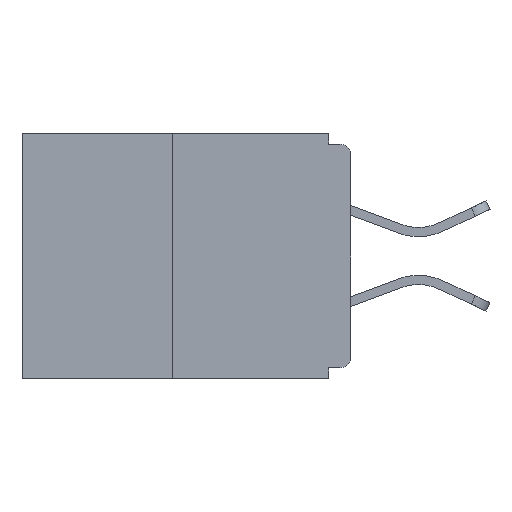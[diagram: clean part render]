
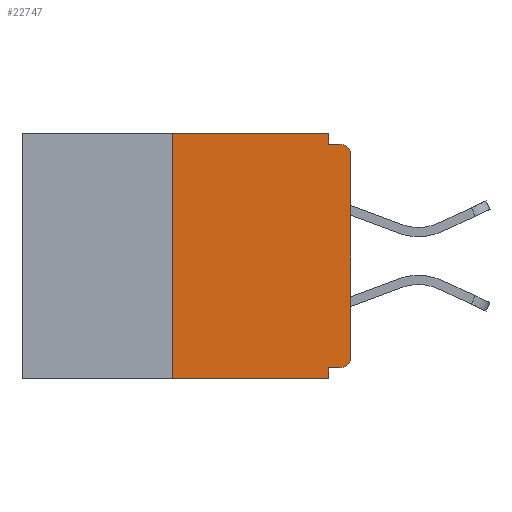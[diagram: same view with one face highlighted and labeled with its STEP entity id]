
A CAD part, left-side view. The second image highlights one B-rep face of the part: STEP entity #22747.
In plain terms, the highlighted planar face has unit normal (-1, 0, 0).
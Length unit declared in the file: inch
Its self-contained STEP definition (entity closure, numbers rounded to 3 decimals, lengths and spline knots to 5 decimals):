
#349 = EDGE_CURVE ( 'NONE', #19427, #4706, #14187, .T. ) ;
#406 = VECTOR ( 'NONE', #24897, 39.37008 ) ;
#541 = DIRECTION ( 'NONE',  ( 0., 0., -1. ) ) ;
#572 = EDGE_CURVE ( 'NONE', #20106, #1014, #22876, .T. ) ;
#596 = CARTESIAN_POINT ( 'NONE',  ( 0., 0., -0.015 ) ) ;
#1014 = VERTEX_POINT ( 'NONE', #19619 ) ;
#1073 = CARTESIAN_POINT ( 'NONE',  ( 0., 0., -0.328 ) ) ;
#1131 = CARTESIAN_POINT ( 'NONE',  ( 0., 0.46, 0. ) ) ;
#1198 = VECTOR ( 'NONE', #21875, 39.37008 ) ;
#1349 = LINE ( 'NONE', #25232, #16736 ) ;
#1517 = DIRECTION ( 'NONE',  ( 0., 0., 1. ) ) ;
#1819 = ORIENTED_EDGE ( 'NONE', *, *, #2468, .T. ) ;
#2040 = CARTESIAN_POINT ( 'NONE',  ( 0., 0.46, -0.343 ) ) ;
#2235 = CARTESIAN_POINT ( 'NONE',  ( 0., 0.031, -0.015 ) ) ;
#2468 = EDGE_CURVE ( 'NONE', #14985, #15072, #26437, .T. ) ;
#2752 = DIRECTION ( 'NONE',  ( 1., 0., 0. ) ) ;
#3038 = EDGE_CURVE ( 'NONE', #20106, #19427, #1349, .T. ) ;
#3979 = VERTEX_POINT ( 'NONE', #15724 ) ;
#4272 = PLANE ( 'NONE',  #24628 ) ;
#4290 = ORIENTED_EDGE ( 'NONE', *, *, #21167, .F. ) ;
#4447 = CIRCLE ( 'NONE', #7449, 0.015 ) ;
#4706 = VERTEX_POINT ( 'NONE', #12124 ) ;
#4926 = ORIENTED_EDGE ( 'NONE', *, *, #26650, .F. ) ;
#5053 = ORIENTED_EDGE ( 'NONE', *, *, #13927, .F. ) ;
#5504 = DIRECTION ( 'NONE',  ( 0., 0., -1. ) ) ;
#6640 = CARTESIAN_POINT ( 'NONE',  ( 0., 0.031, -0.328 ) ) ;
#6810 = DIRECTION ( 'NONE',  ( 0., 0., -1. ) ) ;
#6974 = ORIENTED_EDGE ( 'NONE', *, *, #572, .T. ) ;
#7228 = DIRECTION ( 'NONE',  ( 0., 1., 0. ) ) ;
#7261 = VECTOR ( 'NONE', #541, 39.37008 ) ;
#7382 = DIRECTION ( 'NONE',  ( 0., 0., -1. ) ) ;
#7449 = AXIS2_PLACEMENT_3D ( 'NONE', #15777, #21948, #7382 ) ;
#7498 = VERTEX_POINT ( 'NONE', #6640 ) ;
#8123 = EDGE_LOOP ( 'NONE', ( #26957, #25000, #6974, #15115, #4290, #11863, #1819, #8735, #4926, #5053 ) ) ;
#8735 = ORIENTED_EDGE ( 'NONE', *, *, #22534, .T. ) ;
#8848 = CARTESIAN_POINT ( 'NONE',  ( 0., 0.031, 0. ) ) ;
#9952 = CARTESIAN_POINT ( 'NONE',  ( 0., 0., 0. ) ) ;
#9956 = VERTEX_POINT ( 'NONE', #2235 ) ;
#10528 = VECTOR ( 'NONE', #7228, 39.37008 ) ;
#10941 = CARTESIAN_POINT ( 'NONE',  ( 0., 0., -0.313 ) ) ;
#11050 = CARTESIAN_POINT ( 'NONE',  ( 0., 0.25, 0. ) ) ;
#11109 = CIRCLE ( 'NONE', #16360, 0.015 ) ;
#11243 = EDGE_CURVE ( 'NONE', #27666, #14985, #11109, .T. ) ;
#11863 = ORIENTED_EDGE ( 'NONE', *, *, #11243, .T. ) ;
#12124 = CARTESIAN_POINT ( 'NONE',  ( 0., 0.031, 0. ) ) ;
#12838 = VECTOR ( 'NONE', #25563, 39.37008 ) ;
#12874 = LINE ( 'NONE', #596, #1198 ) ;
#13694 = CARTESIAN_POINT ( 'NONE',  ( 0., 0.015, -0.313 ) ) ;
#13927 = EDGE_CURVE ( 'NONE', #4706, #9956, #16275, .T. ) ;
#14187 = LINE ( 'NONE', #1131, #21891 ) ;
#14985 = VERTEX_POINT ( 'NONE', #10941 ) ;
#15072 = VERTEX_POINT ( 'NONE', #19810 ) ;
#15115 = ORIENTED_EDGE ( 'NONE', *, *, #16617, .F. ) ;
#15559 = CARTESIAN_POINT ( 'NONE',  ( 0., 0.46, 0. ) ) ;
#15724 = CARTESIAN_POINT ( 'NONE',  ( 0., 0.015, -0.015 ) ) ;
#15758 = DIRECTION ( 'NONE',  ( -1., 0., 0. ) ) ;
#15777 = CARTESIAN_POINT ( 'NONE',  ( 0., 0.015, -0.03 ) ) ;
#15841 = DIRECTION ( 'NONE',  ( 0., 0., -1. ) ) ;
#16126 = DIRECTION ( 'NONE',  ( 0., -1., 0. ) ) ;
#16275 = LINE ( 'NONE', #8848, #7261 ) ;
#16360 = AXIS2_PLACEMENT_3D ( 'NONE', #13694, #15758, #5504 ) ;
#16617 = EDGE_CURVE ( 'NONE', #7498, #1014, #25521, .T. ) ;
#16736 = VECTOR ( 'NONE', #1517, 39.37008 ) ;
#19427 = VERTEX_POINT ( 'NONE', #11050 ) ;
#19619 = CARTESIAN_POINT ( 'NONE',  ( 0., 0.031, -0.343 ) ) ;
#19810 = CARTESIAN_POINT ( 'NONE',  ( 0., 0., -0.03 ) ) ;
#20106 = VERTEX_POINT ( 'NONE', #22079 ) ;
#21167 = EDGE_CURVE ( 'NONE', #27666, #7498, #25868, .T. ) ;
#21869 = CARTESIAN_POINT ( 'NONE',  ( 0., 0.015, -0.328 ) ) ;
#21875 = DIRECTION ( 'NONE',  ( 0., -1., 0. ) ) ;
#21891 = VECTOR ( 'NONE', #16126, 39.37008 ) ;
#21948 = DIRECTION ( 'NONE',  ( -1., 0., 0. ) ) ;
#22079 = CARTESIAN_POINT ( 'NONE',  ( 0., 0.25, -0.343 ) ) ;
#22147 = FACE_OUTER_BOUND ( 'NONE', #8123, .T. ) ;
#22170 = VECTOR ( 'NONE', #15841, 39.37008 ) ;
#22534 = EDGE_CURVE ( 'NONE', #15072, #3979, #4447, .T. ) ;
#22747 = ADVANCED_FACE ( 'NONE', ( #22147 ), #4272, .F. ) ;
#22876 = LINE ( 'NONE', #2040, #12838 ) ;
#23822 = CARTESIAN_POINT ( 'NONE',  ( 0., 0.031, -0.343 ) ) ;
#24628 = AXIS2_PLACEMENT_3D ( 'NONE', #15559, #2752, #6810 ) ;
#24897 = DIRECTION ( 'NONE',  ( 0., 0., 1. ) ) ;
#25000 = ORIENTED_EDGE ( 'NONE', *, *, #3038, .F. ) ;
#25232 = CARTESIAN_POINT ( 'NONE',  ( 0., 0.25, 0. ) ) ;
#25521 = LINE ( 'NONE', #23822, #22170 ) ;
#25563 = DIRECTION ( 'NONE',  ( 0., -1., 0. ) ) ;
#25868 = LINE ( 'NONE', #1073, #10528 ) ;
#26437 = LINE ( 'NONE', #9952, #406 ) ;
#26650 = EDGE_CURVE ( 'NONE', #9956, #3979, #12874, .T. ) ;
#26957 = ORIENTED_EDGE ( 'NONE', *, *, #349, .F. ) ;
#27666 = VERTEX_POINT ( 'NONE', #21869 ) ;
